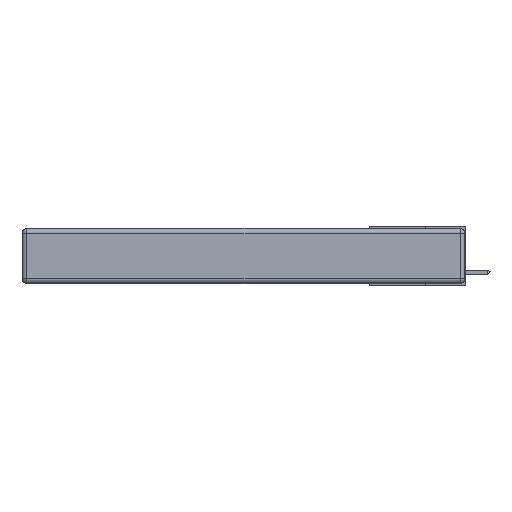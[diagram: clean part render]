
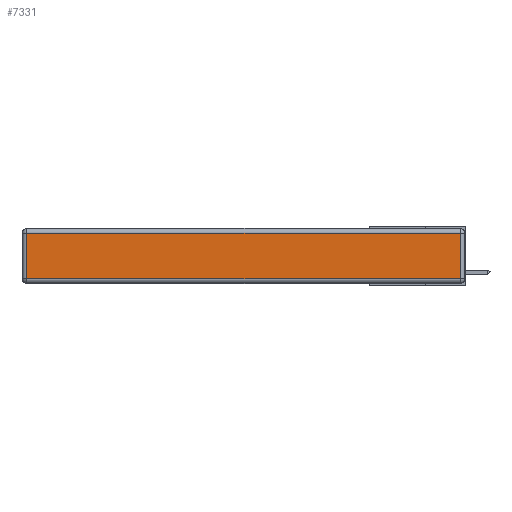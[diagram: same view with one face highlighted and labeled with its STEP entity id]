
A CAD part, left-side view. The second image highlights one B-rep face of the part: STEP entity #7331.
In plain terms, the highlighted planar face has unit normal (-1, 0, 0).
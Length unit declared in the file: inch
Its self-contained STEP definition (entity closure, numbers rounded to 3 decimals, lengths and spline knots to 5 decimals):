
#1165 = AXIS2_PLACEMENT_3D ( 'NONE', #21908, #23924, #15932 ) ;
#2052 = CARTESIAN_POINT ( 'NONE',  ( 0., 2.75, -0.03 ) ) ;
#2159 = CARTESIAN_POINT ( 'NONE',  ( 0., 0.03, -0.343 ) ) ;
#2328 = DIRECTION ( 'NONE',  ( 0., 0., 1. ) ) ;
#3166 = VERTEX_POINT ( 'NONE', #21699 ) ;
#6743 = LINE ( 'NONE', #2159, #15225 ) ;
#6880 = VECTOR ( 'NONE', #24984, 39.37008 ) ;
#6894 = VECTOR ( 'NONE', #8061, 39.37008 ) ;
#7331 = ADVANCED_FACE ( 'NONE', ( #21670 ), #13459, .T. ) ;
#7992 = EDGE_CURVE ( 'NONE', #3166, #18103, #16913, .T. ) ;
#8061 = DIRECTION ( 'NONE',  ( 0., 1., 0. ) ) ;
#8887 = LINE ( 'NONE', #25738, #18643 ) ;
#9697 = DIRECTION ( 'NONE',  ( 0., 0., -1. ) ) ;
#12566 = ORIENTED_EDGE ( 'NONE', *, *, #17240, .T. ) ;
#12675 = CARTESIAN_POINT ( 'NONE',  ( 0., 0.03, -0.313 ) ) ;
#12693 = VERTEX_POINT ( 'NONE', #18684 ) ;
#13459 = PLANE ( 'NONE',  #1165 ) ;
#15225 = VECTOR ( 'NONE', #2328, 39.37008 ) ;
#15932 = DIRECTION ( 'NONE',  ( 0., 0., 1. ) ) ;
#16913 = LINE ( 'NONE', #20969, #6880 ) ;
#17216 = VERTEX_POINT ( 'NONE', #24291 ) ;
#17240 = EDGE_CURVE ( 'NONE', #12693, #17216, #21027, .T. ) ;
#18103 = VERTEX_POINT ( 'NONE', #12675 ) ;
#18643 = VECTOR ( 'NONE', #9697, 39.37008 ) ;
#18684 = CARTESIAN_POINT ( 'NONE',  ( 0., 0.03, -0.03 ) ) ;
#19459 = EDGE_CURVE ( 'NONE', #18103, #12693, #6743, .T. ) ;
#20201 = EDGE_CURVE ( 'NONE', #17216, #3166, #8887, .T. ) ;
#20969 = CARTESIAN_POINT ( 'NONE',  ( 0., 0., -0.313 ) ) ;
#21027 = LINE ( 'NONE', #2052, #6894 ) ;
#21670 = FACE_OUTER_BOUND ( 'NONE', #22658, .T. ) ;
#21699 = CARTESIAN_POINT ( 'NONE',  ( 0., 2.72, -0.313 ) ) ;
#21908 = CARTESIAN_POINT ( 'NONE',  ( 0., 0., -0.343 ) ) ;
#22050 = ORIENTED_EDGE ( 'NONE', *, *, #20201, .T. ) ;
#22658 = EDGE_LOOP ( 'NONE', ( #23092, #25847, #12566, #22050 ) ) ;
#23092 = ORIENTED_EDGE ( 'NONE', *, *, #7992, .T. ) ;
#23924 = DIRECTION ( 'NONE',  ( -1., 0., 0. ) ) ;
#24291 = CARTESIAN_POINT ( 'NONE',  ( 0., 2.72, -0.03 ) ) ;
#24984 = DIRECTION ( 'NONE',  ( 0., -1., 0. ) ) ;
#25738 = CARTESIAN_POINT ( 'NONE',  ( 0., 2.72, -0.343 ) ) ;
#25847 = ORIENTED_EDGE ( 'NONE', *, *, #19459, .T. ) ;
